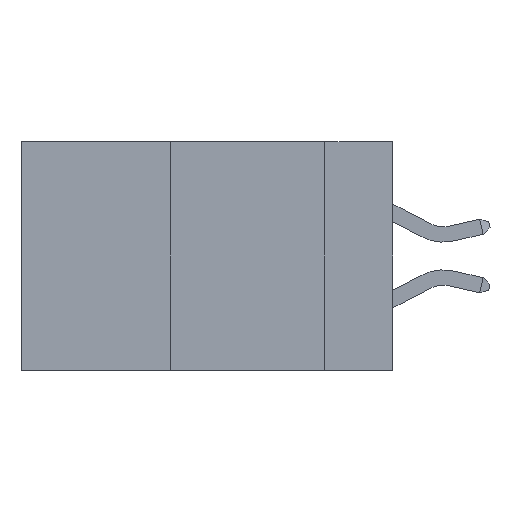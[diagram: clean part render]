
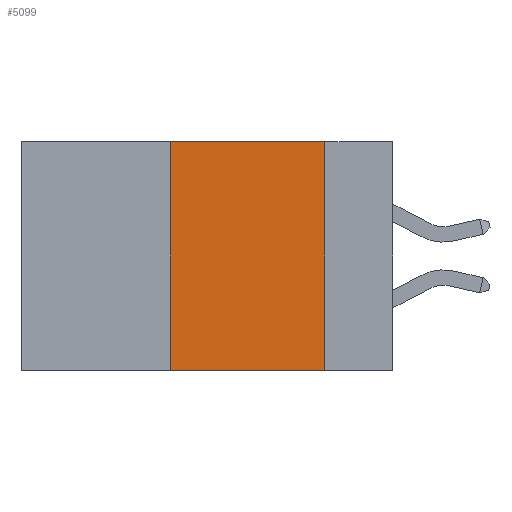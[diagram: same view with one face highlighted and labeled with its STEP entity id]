
A CAD part, left-side view. The second image highlights one B-rep face of the part: STEP entity #5099.
In plain terms, the highlighted planar face has unit normal (-1, 0, 0).
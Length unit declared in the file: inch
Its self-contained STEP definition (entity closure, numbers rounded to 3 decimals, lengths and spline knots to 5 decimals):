
#65 = DIRECTION ( 'NONE',  ( 0., -1., 0. ) ) ;
#143 = EDGE_CURVE ( 'NONE', #1102, #8697, #8256, .T. ) ;
#240 = CARTESIAN_POINT ( 'NONE',  ( 0., 0.36, 0. ) ) ;
#311 = LINE ( 'NONE', #5675, #2967 ) ;
#671 = EDGE_LOOP ( 'NONE', ( #14614, #16445, #11766, #1000 ) ) ;
#987 = EDGE_CURVE ( 'NONE', #17341, #7207, #311, .T. ) ;
#1000 = ORIENTED_EDGE ( 'NONE', *, *, #987, .T. ) ;
#1102 = VERTEX_POINT ( 'NONE', #1986 ) ;
#1374 = DIRECTION ( 'NONE',  ( 0., -1., 0. ) ) ;
#1394 = AXIS2_PLACEMENT_3D ( 'NONE', #10855, #2891, #2803 ) ;
#1724 = EDGE_CURVE ( 'NONE', #17341, #1102, #15288, .T. ) ;
#1739 = DIRECTION ( 'NONE',  ( 0., 0., 1. ) ) ;
#1986 = CARTESIAN_POINT ( 'NONE',  ( 0., 0.36, 0. ) ) ;
#2061 = DIRECTION ( 'NONE',  ( 0., 0., -1. ) ) ;
#2803 = DIRECTION ( 'NONE',  ( 0., 0., -1. ) ) ;
#2891 = DIRECTION ( 'NONE',  ( 1., 0., 0. ) ) ;
#2965 = CARTESIAN_POINT ( 'NONE',  ( 0., 0.11, 0. ) ) ;
#2967 = VECTOR ( 'NONE', #1374, 39.37008 ) ;
#4242 = EDGE_CURVE ( 'NONE', #8697, #7207, #12848, .T. ) ;
#4373 = CARTESIAN_POINT ( 'NONE',  ( 0., 0.6, 0. ) ) ;
#5099 = ADVANCED_FACE ( 'NONE', ( #15024 ), #6783, .F. ) ;
#5675 = CARTESIAN_POINT ( 'NONE',  ( 0., 0.6, -0.37 ) ) ;
#6783 = PLANE ( 'NONE',  #1394 ) ;
#7207 = VERTEX_POINT ( 'NONE', #10564 ) ;
#8256 = LINE ( 'NONE', #4373, #12831 ) ;
#8656 = CARTESIAN_POINT ( 'NONE',  ( 0., 0.11, 0. ) ) ;
#8697 = VERTEX_POINT ( 'NONE', #2965 ) ;
#10564 = CARTESIAN_POINT ( 'NONE',  ( 0., 0.11, -0.37 ) ) ;
#10855 = CARTESIAN_POINT ( 'NONE',  ( 0., 0.6, 0. ) ) ;
#11766 = ORIENTED_EDGE ( 'NONE', *, *, #1724, .F. ) ;
#11795 = VECTOR ( 'NONE', #1739, 39.37008 ) ;
#12831 = VECTOR ( 'NONE', #65, 39.37008 ) ;
#12848 = LINE ( 'NONE', #8656, #13224 ) ;
#13224 = VECTOR ( 'NONE', #2061, 39.37008 ) ;
#14614 = ORIENTED_EDGE ( 'NONE', *, *, #4242, .F. ) ;
#14716 = CARTESIAN_POINT ( 'NONE',  ( 0., 0.36, -0.37 ) ) ;
#15024 = FACE_OUTER_BOUND ( 'NONE', #671, .T. ) ;
#15288 = LINE ( 'NONE', #240, #11795 ) ;
#16445 = ORIENTED_EDGE ( 'NONE', *, *, #143, .F. ) ;
#17341 = VERTEX_POINT ( 'NONE', #14716 ) ;
